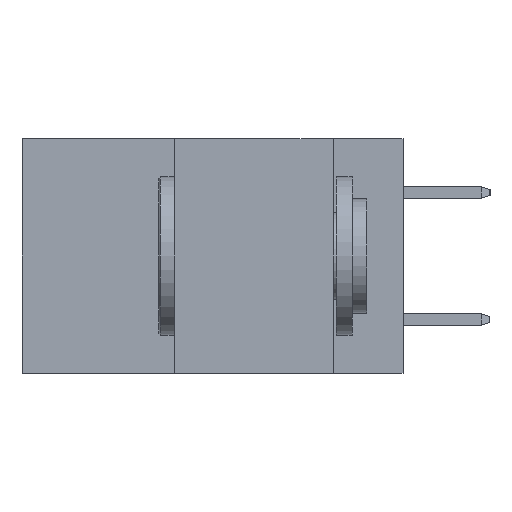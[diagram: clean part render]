
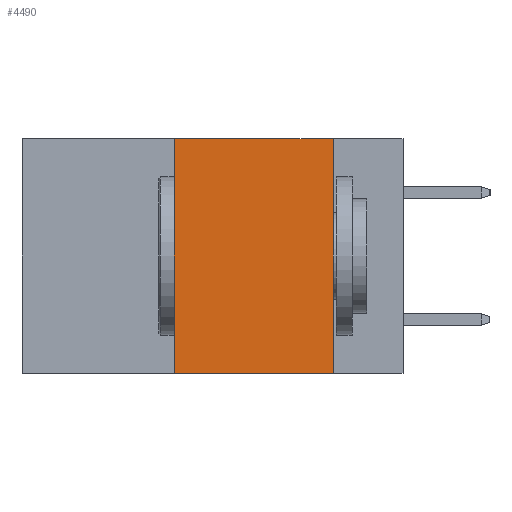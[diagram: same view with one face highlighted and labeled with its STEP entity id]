
A CAD part, left-side view. The second image highlights one B-rep face of the part: STEP entity #4490.
In plain terms, the highlighted planar face has unit normal (-1, 0, 0).
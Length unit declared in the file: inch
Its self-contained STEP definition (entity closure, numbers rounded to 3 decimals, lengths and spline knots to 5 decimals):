
#952 = VERTEX_POINT ( 'NONE', #44549 ) ;
#1301 = LINE ( 'NONE', #30928, #15060 ) ;
#3037 = VERTEX_POINT ( 'NONE', #22878 ) ;
#4397 = VERTEX_POINT ( 'NONE', #18440 ) ;
#4490 = ADVANCED_FACE ( 'NONE', ( #5123 ), #34058, .F. ) ;
#4691 = EDGE_CURVE ( 'NONE', #4397, #952, #39247, .T. ) ;
#4741 = ORIENTED_EDGE ( 'NONE', *, *, #4691, .F. ) ;
#5027 = CARTESIAN_POINT ( 'NONE',  ( 0., 0.36, -0.37 ) ) ;
#5123 = FACE_OUTER_BOUND ( 'NONE', #20439, .T. ) ;
#5526 = EDGE_CURVE ( 'NONE', #952, #3037, #6590, .T. ) ;
#5612 = CARTESIAN_POINT ( 'NONE',  ( 0., 0.36, 0. ) ) ;
#5826 = CARTESIAN_POINT ( 'NONE',  ( 0., 0.6, 0. ) ) ;
#6590 = LINE ( 'NONE', #39317, #8847 ) ;
#8847 = VECTOR ( 'NONE', #35983, 39.37008 ) ;
#12011 = EDGE_CURVE ( 'NONE', #30977, #3037, #1301, .T. ) ;
#12720 = CARTESIAN_POINT ( 'NONE',  ( 0., 0.6, 0. ) ) ;
#15060 = VECTOR ( 'NONE', #19794, 39.37008 ) ;
#18440 = CARTESIAN_POINT ( 'NONE',  ( 0., 0.36, 0. ) ) ;
#19794 = DIRECTION ( 'NONE',  ( 0., -1., 0. ) ) ;
#20439 = EDGE_LOOP ( 'NONE', ( #41163, #4741, #45776, #39187 ) ) ;
#22276 = EDGE_CURVE ( 'NONE', #30977, #4397, #38573, .T. ) ;
#22878 = CARTESIAN_POINT ( 'NONE',  ( 0., 0.11, -0.37 ) ) ;
#30928 = CARTESIAN_POINT ( 'NONE',  ( 0., 0.6, -0.37 ) ) ;
#30977 = VERTEX_POINT ( 'NONE', #5027 ) ;
#33823 = DIRECTION ( 'NONE',  ( 1., 0., 0. ) ) ;
#34058 = PLANE ( 'NONE',  #40250 ) ;
#34785 = DIRECTION ( 'NONE',  ( 0., 0., 1. ) ) ;
#35221 = DIRECTION ( 'NONE',  ( 0., -1., 0. ) ) ;
#35983 = DIRECTION ( 'NONE',  ( 0., 0., -1. ) ) ;
#37389 = DIRECTION ( 'NONE',  ( 0., 0., -1. ) ) ;
#38573 = LINE ( 'NONE', #5612, #40459 ) ;
#39187 = ORIENTED_EDGE ( 'NONE', *, *, #12011, .T. ) ;
#39247 = LINE ( 'NONE', #5826, #41569 ) ;
#39317 = CARTESIAN_POINT ( 'NONE',  ( 0., 0.11, 0. ) ) ;
#40250 = AXIS2_PLACEMENT_3D ( 'NONE', #12720, #33823, #37389 ) ;
#40459 = VECTOR ( 'NONE', #34785, 39.37008 ) ;
#41163 = ORIENTED_EDGE ( 'NONE', *, *, #5526, .F. ) ;
#41569 = VECTOR ( 'NONE', #35221, 39.37008 ) ;
#44549 = CARTESIAN_POINT ( 'NONE',  ( 0., 0.11, 0. ) ) ;
#45776 = ORIENTED_EDGE ( 'NONE', *, *, #22276, .F. ) ;
